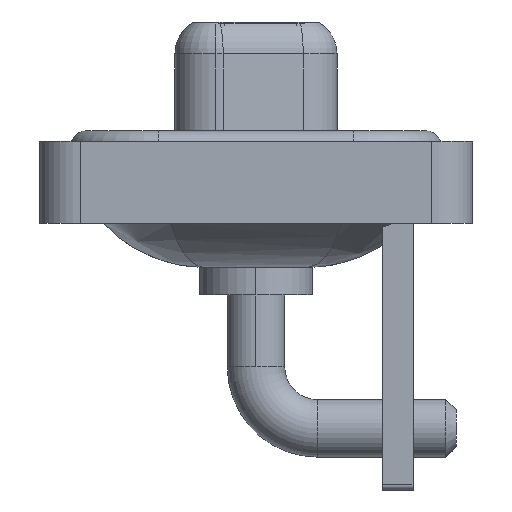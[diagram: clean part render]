
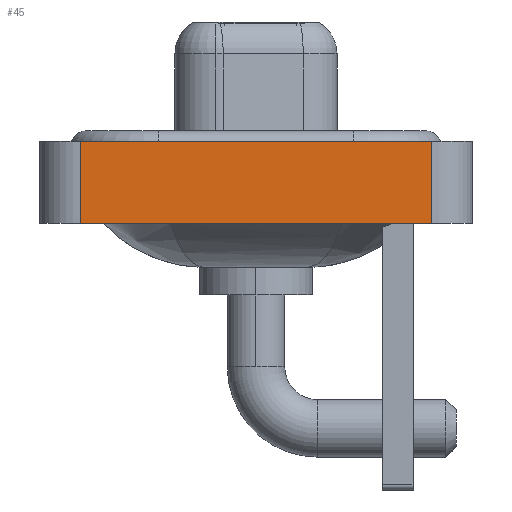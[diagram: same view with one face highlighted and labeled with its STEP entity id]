
A CAD part, left-side view. The second image highlights one B-rep face of the part: STEP entity #45.
In plain terms, the highlighted planar face has unit normal (-1, 0, 0).
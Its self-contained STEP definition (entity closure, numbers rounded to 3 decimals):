
#45 = ADVANCED_FACE ( 'NONE', ( #12966 ), #16652, .T. ) ;
#789 = CARTESIAN_POINT ( 'NONE',  ( -7.3, -8.55, -3.6 ) ) ;
#1494 = CARTESIAN_POINT ( 'NONE',  ( -7.3, 8.55, -3.6 ) ) ;
#1885 = AXIS2_PLACEMENT_3D ( 'NONE', #6521, #8960, #14173 ) ;
#2364 = CARTESIAN_POINT ( 'NONE',  ( -7.3, -8.55, 0.4 ) ) ;
#2563 = ORIENTED_EDGE ( 'NONE', *, *, #9669, .F. ) ;
#3748 = DIRECTION ( 'NONE',  ( 0., 0., 1. ) ) ;
#5237 = LINE ( 'NONE', #11606, #12798 ) ;
#5395 = VECTOR ( 'NONE', #3748, 1000. ) ;
#5954 = VERTEX_POINT ( 'NONE', #9294 ) ;
#6052 = DIRECTION ( 'NONE',  ( 0., -1., 0. ) ) ;
#6468 = LINE ( 'NONE', #1494, #5395 ) ;
#6521 = CARTESIAN_POINT ( 'NONE',  ( -7.3, -8.55, -3.6 ) ) ;
#6676 = VECTOR ( 'NONE', #6052, 1000. ) ;
#7709 = VERTEX_POINT ( 'NONE', #2364 ) ;
#8960 = DIRECTION ( 'NONE',  ( -1., 0., 0. ) ) ;
#9183 = ORIENTED_EDGE ( 'NONE', *, *, #10866, .T. ) ;
#9294 = CARTESIAN_POINT ( 'NONE',  ( -7.3, -8.55, -3.6 ) ) ;
#9669 = EDGE_CURVE ( 'NONE', #16465, #15374, #6468, .T. ) ;
#10866 = EDGE_CURVE ( 'NONE', #16465, #5954, #11146, .T. ) ;
#11146 = LINE ( 'NONE', #789, #6676 ) ;
#11606 = CARTESIAN_POINT ( 'NONE',  ( -7.3, -8.55, -3.6 ) ) ;
#11631 = DIRECTION ( 'NONE',  ( 0., -1., 0. ) ) ;
#11889 = CARTESIAN_POINT ( 'NONE',  ( -7.3, -8.55, 0.4 ) ) ;
#12798 = VECTOR ( 'NONE', #16740, 1000. ) ;
#12966 = FACE_OUTER_BOUND ( 'NONE', #15420, .T. ) ;
#13535 = ORIENTED_EDGE ( 'NONE', *, *, #15300, .F. ) ;
#14118 = CARTESIAN_POINT ( 'NONE',  ( -7.3, 8.55, 0.4 ) ) ;
#14173 = DIRECTION ( 'NONE',  ( 0., 0., 1. ) ) ;
#14199 = LINE ( 'NONE', #11889, #14997 ) ;
#14997 = VECTOR ( 'NONE', #11631, 1000. ) ;
#15300 = EDGE_CURVE ( 'NONE', #15374, #7709, #14199, .T. ) ;
#15374 = VERTEX_POINT ( 'NONE', #14118 ) ;
#15420 = EDGE_LOOP ( 'NONE', ( #15829, #13535, #2563, #9183 ) ) ;
#15612 = EDGE_CURVE ( 'NONE', #5954, #7709, #5237, .T. ) ;
#15829 = ORIENTED_EDGE ( 'NONE', *, *, #15612, .T. ) ;
#16465 = VERTEX_POINT ( 'NONE', #16553 ) ;
#16553 = CARTESIAN_POINT ( 'NONE',  ( -7.3, 8.55, -3.6 ) ) ;
#16652 = PLANE ( 'NONE',  #1885 ) ;
#16740 = DIRECTION ( 'NONE',  ( 0., 0., 1. ) ) ;
